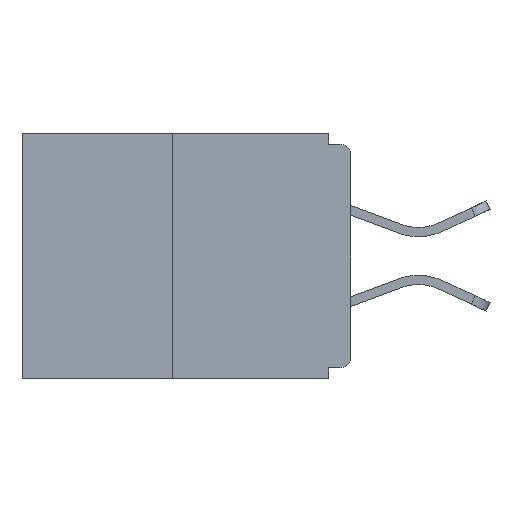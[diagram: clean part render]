
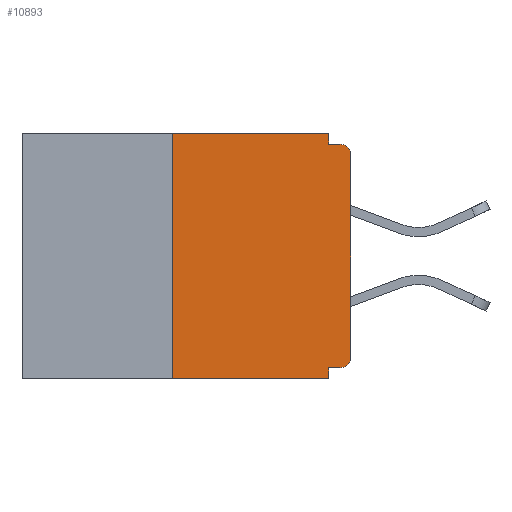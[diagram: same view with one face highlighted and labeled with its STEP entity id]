
A CAD part, left-side view. The second image highlights one B-rep face of the part: STEP entity #10893.
In plain terms, the highlighted planar face has unit normal (-1, 0, 0).
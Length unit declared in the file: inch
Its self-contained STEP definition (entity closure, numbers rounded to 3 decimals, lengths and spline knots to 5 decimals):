
#400 = EDGE_CURVE ( 'NONE', #7371, #5961, #8536, .T. ) ;
#527 = DIRECTION ( 'NONE',  ( 0., 0., -1. ) ) ;
#597 = EDGE_CURVE ( 'NONE', #1427, #3566, #9165, .T. ) ;
#777 = EDGE_CURVE ( 'NONE', #5961, #11115, #13001, .T. ) ;
#972 = DIRECTION ( 'NONE',  ( 0., -1., 0. ) ) ;
#1048 = VECTOR ( 'NONE', #4467, 39.37008 ) ;
#1253 = FACE_OUTER_BOUND ( 'NONE', #8385, .T. ) ;
#1340 = DIRECTION ( 'NONE',  ( 0., 0., -1. ) ) ;
#1427 = VERTEX_POINT ( 'NONE', #1893 ) ;
#1429 = AXIS2_PLACEMENT_3D ( 'NONE', #4098, #11326, #5176 ) ;
#1893 = CARTESIAN_POINT ( 'NONE',  ( 0., 0.031, -0.328 ) ) ;
#2030 = EDGE_CURVE ( 'NONE', #2290, #2116, #4288, .T. ) ;
#2116 = VERTEX_POINT ( 'NONE', #9365 ) ;
#2290 = VERTEX_POINT ( 'NONE', #3744 ) ;
#2330 = VECTOR ( 'NONE', #13080, 39.37008 ) ;
#2420 = CARTESIAN_POINT ( 'NONE',  ( 0., 0.031, -0.015 ) ) ;
#2606 = ORIENTED_EDGE ( 'NONE', *, *, #5807, .F. ) ;
#2688 = AXIS2_PLACEMENT_3D ( 'NONE', #10380, #11464, #8679 ) ;
#2887 = VECTOR ( 'NONE', #5742, 39.37008 ) ;
#3213 = VECTOR ( 'NONE', #7901, 39.37008 ) ;
#3542 = VERTEX_POINT ( 'NONE', #2420 ) ;
#3566 = VERTEX_POINT ( 'NONE', #10456 ) ;
#3581 = DIRECTION ( 'NONE',  ( 1., 0., 0. ) ) ;
#3744 = CARTESIAN_POINT ( 'NONE',  ( 0., 0.25, -0.343 ) ) ;
#3837 = PLANE ( 'NONE',  #8960 ) ;
#3841 = CARTESIAN_POINT ( 'NONE',  ( 0., 0., 0. ) ) ;
#3843 = VERTEX_POINT ( 'NONE', #7105 ) ;
#4098 = CARTESIAN_POINT ( 'NONE',  ( 0., 0.015, -0.03 ) ) ;
#4114 = CARTESIAN_POINT ( 'NONE',  ( 0., 0., -0.015 ) ) ;
#4288 = LINE ( 'NONE', #8243, #5102 ) ;
#4327 = VECTOR ( 'NONE', #1340, 39.37008 ) ;
#4467 = DIRECTION ( 'NONE',  ( 0., 1., 0. ) ) ;
#5058 = LINE ( 'NONE', #6810, #2330 ) ;
#5067 = EDGE_CURVE ( 'NONE', #2290, #3566, #10053, .T. ) ;
#5102 = VECTOR ( 'NONE', #13203, 39.37008 ) ;
#5176 = DIRECTION ( 'NONE',  ( 0., 0., -1. ) ) ;
#5742 = DIRECTION ( 'NONE',  ( 0., -1., 0. ) ) ;
#5807 = EDGE_CURVE ( 'NONE', #7371, #1427, #9561, .T. ) ;
#5961 = VERTEX_POINT ( 'NONE', #10718 ) ;
#6214 = ORIENTED_EDGE ( 'NONE', *, *, #5067, .T. ) ;
#6222 = CARTESIAN_POINT ( 'NONE',  ( 0., 0.031, 0. ) ) ;
#6260 = ORIENTED_EDGE ( 'NONE', *, *, #8231, .F. ) ;
#6302 = ORIENTED_EDGE ( 'NONE', *, *, #777, .T. ) ;
#6380 = VECTOR ( 'NONE', #972, 39.37008 ) ;
#6408 = ORIENTED_EDGE ( 'NONE', *, *, #597, .F. ) ;
#6486 = ORIENTED_EDGE ( 'NONE', *, *, #2030, .F. ) ;
#6717 = CARTESIAN_POINT ( 'NONE',  ( 0., 0.46, 0. ) ) ;
#6810 = CARTESIAN_POINT ( 'NONE',  ( 0., 0.031, 0. ) ) ;
#7105 = CARTESIAN_POINT ( 'NONE',  ( 0., 0.015, -0.015 ) ) ;
#7168 = ORIENTED_EDGE ( 'NONE', *, *, #12038, .F. ) ;
#7371 = VERTEX_POINT ( 'NONE', #10951 ) ;
#7564 = CARTESIAN_POINT ( 'NONE',  ( 0., 0.031, -0.343 ) ) ;
#7901 = DIRECTION ( 'NONE',  ( 0., 0., 1. ) ) ;
#8231 = EDGE_CURVE ( 'NONE', #3542, #3843, #9495, .T. ) ;
#8243 = CARTESIAN_POINT ( 'NONE',  ( 0., 0.25, 0. ) ) ;
#8385 = EDGE_LOOP ( 'NONE', ( #12612, #6486, #6214, #6408, #2606, #12239, #6302, #11149, #6260, #7168 ) ) ;
#8452 = DIRECTION ( 'NONE',  ( 0., -1., 0. ) ) ;
#8536 = CIRCLE ( 'NONE', #2688, 0.015 ) ;
#8575 = CIRCLE ( 'NONE', #1429, 0.015 ) ;
#8672 = EDGE_CURVE ( 'NONE', #2116, #11485, #12383, .T. ) ;
#8679 = DIRECTION ( 'NONE',  ( 0., 0., -1. ) ) ;
#8960 = AXIS2_PLACEMENT_3D ( 'NONE', #11854, #3581, #527 ) ;
#9165 = LINE ( 'NONE', #7564, #4327 ) ;
#9365 = CARTESIAN_POINT ( 'NONE',  ( 0., 0.25, 0. ) ) ;
#9495 = LINE ( 'NONE', #4114, #9965 ) ;
#9561 = LINE ( 'NONE', #10628, #1048 ) ;
#9965 = VECTOR ( 'NONE', #8452, 39.37008 ) ;
#10053 = LINE ( 'NONE', #10146, #6380 ) ;
#10146 = CARTESIAN_POINT ( 'NONE',  ( 0., 0.46, -0.343 ) ) ;
#10380 = CARTESIAN_POINT ( 'NONE',  ( 0., 0.015, -0.313 ) ) ;
#10456 = CARTESIAN_POINT ( 'NONE',  ( 0., 0.031, -0.343 ) ) ;
#10628 = CARTESIAN_POINT ( 'NONE',  ( 0., 0., -0.328 ) ) ;
#10718 = CARTESIAN_POINT ( 'NONE',  ( 0., 0., -0.313 ) ) ;
#10893 = ADVANCED_FACE ( 'NONE', ( #1253 ), #3837, .F. ) ;
#10951 = CARTESIAN_POINT ( 'NONE',  ( 0., 0.015, -0.328 ) ) ;
#11115 = VERTEX_POINT ( 'NONE', #11680 ) ;
#11149 = ORIENTED_EDGE ( 'NONE', *, *, #12916, .T. ) ;
#11326 = DIRECTION ( 'NONE',  ( -1., 0., 0. ) ) ;
#11464 = DIRECTION ( 'NONE',  ( -1., 0., 0. ) ) ;
#11485 = VERTEX_POINT ( 'NONE', #6222 ) ;
#11680 = CARTESIAN_POINT ( 'NONE',  ( 0., 0., -0.03 ) ) ;
#11854 = CARTESIAN_POINT ( 'NONE',  ( 0., 0.46, 0. ) ) ;
#12038 = EDGE_CURVE ( 'NONE', #11485, #3542, #5058, .T. ) ;
#12239 = ORIENTED_EDGE ( 'NONE', *, *, #400, .T. ) ;
#12383 = LINE ( 'NONE', #6717, #2887 ) ;
#12612 = ORIENTED_EDGE ( 'NONE', *, *, #8672, .F. ) ;
#12916 = EDGE_CURVE ( 'NONE', #11115, #3843, #8575, .T. ) ;
#13001 = LINE ( 'NONE', #3841, #3213 ) ;
#13080 = DIRECTION ( 'NONE',  ( 0., 0., -1. ) ) ;
#13203 = DIRECTION ( 'NONE',  ( 0., 0., 1. ) ) ;
